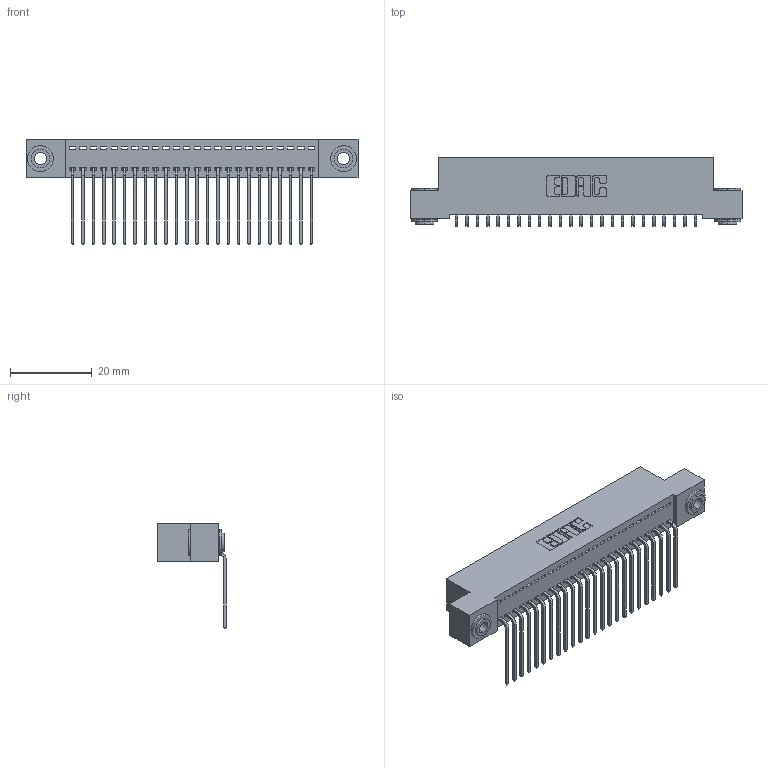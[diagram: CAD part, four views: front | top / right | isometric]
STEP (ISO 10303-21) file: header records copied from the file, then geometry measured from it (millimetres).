
FILE_DESCRIPTION (( 'STEP AP203' ), '1' );
FILE_NAME ('342-024-559-103.STEP', '2019-10-02T00:16:55', ( '' ), ( '' ), 'SwSTEP 2.0', 'SolidWorks 2016', '' );
FILE_SCHEMA (( 'CONFIG_CONTROL_DESIGN' ));
Length unit declared in the file: inch
Products named in the file (4): 342 Part_.156 TH; 345-292-001_558 559 Tail - 1; 342-250-002_345-250-002-102; 342-024-559-103
Assembly tree (27 placements, depth 2):
  342-024-559-103
    342 Part_.156 TH
    345-292-001_558 559 Tail - 1  x24
    342-250-002_345-250-002-102  x2
Bounding box: 81.28 x 16.83 x 25.78 mm (x, y, z)
Volume: 7163.1 mm3; surface area: 10862.9 mm2
Topology: 27 solids, 27 shells, 1588 faces, 4743 edges, 3126 vertices
Faces by surface type: plane 1132, cylinder 448, cone 8
Entity records: 17602 total; most frequent: CARTESIAN_POINT 3017, ORIENTED_EDGE 2970, DIRECTION 2615, EDGE_CURVE 1485, VECTOR 1333, LINE 1333, VERTEX_POINT 986, AXIS2_PLACEMENT_3D 641
